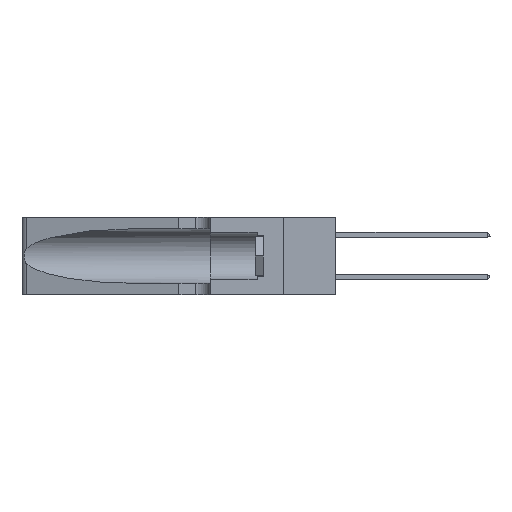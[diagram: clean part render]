
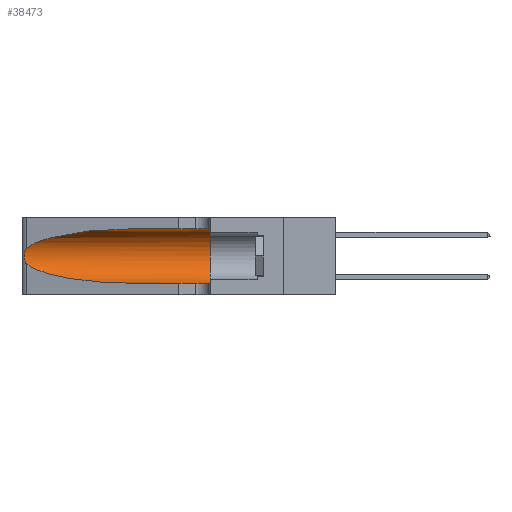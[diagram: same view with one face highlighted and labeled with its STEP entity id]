
A CAD part, left-side view. The second image highlights one B-rep face of the part: STEP entity #38473.
In plain terms, the highlighted cylindrical face has radius 3.308 mm (diameter 6.617 mm), a partial arc.
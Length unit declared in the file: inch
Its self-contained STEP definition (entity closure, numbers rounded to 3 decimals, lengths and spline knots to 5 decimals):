
#90 = CARTESIAN_POINT ( 'NONE',  ( 0.26075, 1.23896, 0.178 ) ) ;
#394 = CARTESIAN_POINT ( 'NONE',  ( 0.2373, 1.15595, 0.28018 ) ) ;
#1600 = VERTEX_POINT ( 'NONE', #12851 ) ;
#2201 = CARTESIAN_POINT ( 'NONE',  ( 0.2373, 1.15595, 0.08982 ) ) ;
#2355 = AXIS2_PLACEMENT_3D ( 'NONE', #10612, #33338, #13877 ) ;
#2603 = EDGE_CURVE ( 'NONE', #1600, #25852, #18470, .T. ) ;
#3330 = CARTESIAN_POINT ( 'NONE',  ( 0.1305, 1.61858, 0.185 ) ) ;
#3460 = CARTESIAN_POINT ( 'NONE',  ( 0.25856, 1.23593, 0.16098 ) ) ;
#5503 = CARTESIAN_POINT ( 'NONE',  ( 0.1305, 0.72297, 0.05475 ) ) ;
#6757 = CARTESIAN_POINT ( 'NONE',  ( 0.25639, 1.23186, 0.15144 ) ) ;
#7555 = CYLINDRICAL_SURFACE ( 'NONE', #35209, 0.13025 ) ;
#8068 = ORIENTED_EDGE ( 'NONE', *, *, #27323, .T. ) ;
#8092 = DIRECTION ( 'NONE',  ( 0., -1., 0. ) ) ;
#8273 =( BOUNDED_CURVE ( )  B_SPLINE_CURVE ( 3, ( #36099, #19930, #394, #23223 ),
 .UNSPECIFIED., .F., .F. ) 
 B_SPLINE_CURVE_WITH_KNOTS ( ( 4, 4 ),
 ( 1.5708, 2.84003 ),
 .UNSPECIFIED. ) 
 CURVE ( )  GEOMETRIC_REPRESENTATION_ITEM ( )  RATIONAL_B_SPLINE_CURVE ( ( 1., 0.87, 0.87, 1. ) ) 
 REPRESENTATION_ITEM ( '' )  );
#8806 = VECTOR ( 'NONE', #8092, 39.37008 ) ;
#9259 = CIRCLE ( 'NONE', #2355, 0.13025 ) ;
#9725 = DIRECTION ( 'NONE',  ( 0., 0., -1. ) ) ;
#9850 = CARTESIAN_POINT ( 'NONE',  ( 0.25487, 1.22718, 0.22369 ) ) ;
#9984 = CARTESIAN_POINT ( 'NONE',  ( 0.25487, 1.22718, 0.14631 ) ) ;
#10612 = CARTESIAN_POINT ( 'NONE',  ( 0.1305, 0.35, 0.185 ) ) ;
#10692 = EDGE_LOOP ( 'NONE', ( #21285, #29918, #23344, #8068, #30453, #32510 ) ) ;
#11349 = CARTESIAN_POINT ( 'NONE',  ( 0.1305, 1.61858, 0.31525 ) ) ;
#12851 = CARTESIAN_POINT ( 'NONE',  ( 0.1305, 0.72297, 0.31525 ) ) ;
#13093 = CARTESIAN_POINT ( 'NONE',  ( 0.25639, 1.23184, 0.21858 ) ) ;
#13877 = DIRECTION ( 'NONE',  ( 0., 0., 1. ) ) ;
#16302 = EDGE_CURVE ( 'NONE', #1600, #18834, #8273, .T. ) ;
#16381 = CARTESIAN_POINT ( 'NONE',  ( 0.25854, 1.2359, 0.20912 ) ) ;
#16649 = CARTESIAN_POINT ( 'NONE',  ( 0.1305, 0.72297, 0.05475 ) ) ;
#16748 = CARTESIAN_POINT ( 'NONE',  ( 0.25487, 1.22718, 0.22369 ) ) ;
#17626 = VERTEX_POINT ( 'NONE', #23523 ) ;
#18470 = LINE ( 'NONE', #11349, #8806 ) ;
#18834 = VERTEX_POINT ( 'NONE', #16748 ) ;
#19647 = CARTESIAN_POINT ( 'NONE',  ( 0.26075, 1.23896, 0.19203 ) ) ;
#19930 = CARTESIAN_POINT ( 'NONE',  ( 0.18966, 0.96281, 0.31525 ) ) ;
#20251 = B_SPLINE_CURVE_WITH_KNOTS ( 'NONE', 3,
 ( #9850, #26051, #13093, #35815, #16381, #39067, #19647, #90, #22937, #3460, #26196, #6757, #29454, #9984 ),
 .UNSPECIFIED., .F., .F.,
 ( 4, 2, 2, 2, 2, 2, 4 ),
 ( 0., 0.00027, 0.00053, 0.00107, 0.0016, 0.00187, 0.00214 ),
 .UNSPECIFIED. ) ;
#20697 = VECTOR ( 'NONE', #39767, 39.37008 ) ;
#21285 = ORIENTED_EDGE ( 'NONE', *, *, #16302, .T. ) ;
#22937 = CARTESIAN_POINT ( 'NONE',  ( 0.26017, 1.23833, 0.17102 ) ) ;
#23223 = CARTESIAN_POINT ( 'NONE',  ( 0.25487, 1.22718, 0.22369 ) ) ;
#23344 = ORIENTED_EDGE ( 'NONE', *, *, #37915, .T. ) ;
#23523 = CARTESIAN_POINT ( 'NONE',  ( 0.25487, 1.22718, 0.14631 ) ) ;
#24955 = CARTESIAN_POINT ( 'NONE',  ( 0.18966, 0.96281, 0.05475 ) ) ;
#25852 = VERTEX_POINT ( 'NONE', #41319 ) ;
#26051 = CARTESIAN_POINT ( 'NONE',  ( 0.25555, 1.22994, 0.2215 ) ) ;
#26066 = DIRECTION ( 'NONE',  ( 0., -1., 0. ) ) ;
#26196 = CARTESIAN_POINT ( 'NONE',  ( 0.25789, 1.23486, 0.15765 ) ) ;
#27323 = EDGE_CURVE ( 'NONE', #30579, #31062, #37914, .T. ) ;
#29454 = CARTESIAN_POINT ( 'NONE',  ( 0.25555, 1.22993, 0.14849 ) ) ;
#29918 = ORIENTED_EDGE ( 'NONE', *, *, #32421, .T. ) ;
#30453 = ORIENTED_EDGE ( 'NONE', *, *, #31355, .F. ) ;
#30579 = VERTEX_POINT ( 'NONE', #16649 ) ;
#31062 = VERTEX_POINT ( 'NONE', #41559 ) ;
#31355 = EDGE_CURVE ( 'NONE', #25852, #31062, #9259, .T. ) ;
#32421 = EDGE_CURVE ( 'NONE', #18834, #17626, #20251, .T. ) ;
#32510 = ORIENTED_EDGE ( 'NONE', *, *, #2603, .F. ) ;
#33338 = DIRECTION ( 'NONE',  ( 0., 1., 0. ) ) ;
#33444 = FACE_OUTER_BOUND ( 'NONE', #10692, .T. ) ;
#35209 = AXIS2_PLACEMENT_3D ( 'NONE', #3330, #26066, #9725 ) ;
#35815 = CARTESIAN_POINT ( 'NONE',  ( 0.25787, 1.23484, 0.2124 ) ) ;
#36099 = CARTESIAN_POINT ( 'NONE',  ( 0.1305, 0.72297, 0.31525 ) ) ;
#36503 = CARTESIAN_POINT ( 'NONE',  ( 0.1305, 1.61858, 0.05475 ) ) ;
#37914 = LINE ( 'NONE', #36503, #20697 ) ;
#37915 = EDGE_CURVE ( 'NONE', #17626, #30579, #39749, .T. ) ;
#38473 = ADVANCED_FACE ( 'NONE', ( #33444 ), #7555, .F. ) ;
#39067 = CARTESIAN_POINT ( 'NONE',  ( 0.26018, 1.23835, 0.19895 ) ) ;
#39749 =( BOUNDED_CURVE ( )  B_SPLINE_CURVE ( 3, ( #41095, #2201, #24955, #5503 ),
 .UNSPECIFIED., .F., .F. ) 
 B_SPLINE_CURVE_WITH_KNOTS ( ( 4, 4 ),
 ( 3.44316, 4.71239 ),
 .UNSPECIFIED. ) 
 CURVE ( )  GEOMETRIC_REPRESENTATION_ITEM ( )  RATIONAL_B_SPLINE_CURVE ( ( 1., 0.87, 0.87, 1. ) ) 
 REPRESENTATION_ITEM ( '' )  );
#39767 = DIRECTION ( 'NONE',  ( 0., -1., 0. ) ) ;
#41095 = CARTESIAN_POINT ( 'NONE',  ( 0.25487, 1.22718, 0.14631 ) ) ;
#41319 = CARTESIAN_POINT ( 'NONE',  ( 0.1305, 0.35, 0.31525 ) ) ;
#41559 = CARTESIAN_POINT ( 'NONE',  ( 0.1305, 0.35, 0.05475 ) ) ;
